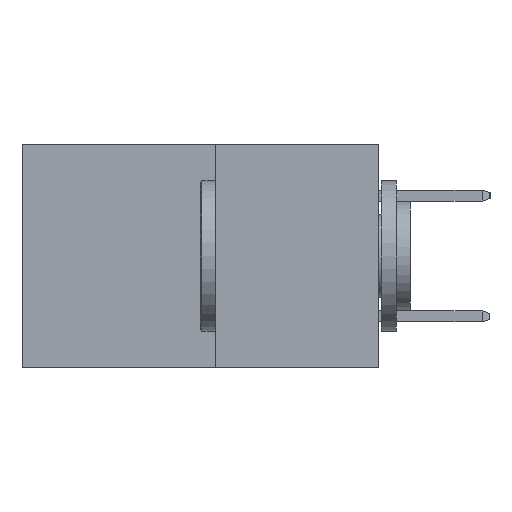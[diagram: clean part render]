
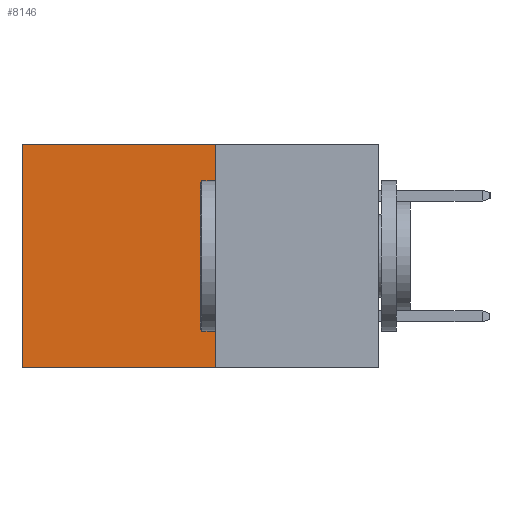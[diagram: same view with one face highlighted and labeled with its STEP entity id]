
A CAD part, left-side view. The second image highlights one B-rep face of the part: STEP entity #8146.
In plain terms, the highlighted planar face has unit normal (-1, 0, 0).
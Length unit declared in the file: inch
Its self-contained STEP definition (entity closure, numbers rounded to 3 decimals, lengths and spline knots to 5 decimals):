
#249 = CARTESIAN_POINT ( 'NONE',  ( 0.277, 0.59, -0.37 ) ) ;
#327 = DIRECTION ( 'NONE',  ( 0., 0., -1. ) ) ;
#389 = EDGE_CURVE ( 'NONE', #13728, #2736, #17457, .T. ) ;
#1051 = DIRECTION ( 'NONE',  ( 0., 1., 0. ) ) ;
#1529 = CARTESIAN_POINT ( 'NONE',  ( 0.277, 0.59, 0. ) ) ;
#1796 = LINE ( 'NONE', #249, #10206 ) ;
#2736 = VERTEX_POINT ( 'NONE', #16507 ) ;
#3475 = FACE_OUTER_BOUND ( 'NONE', #16421, .T. ) ;
#6684 = ORIENTED_EDGE ( 'NONE', *, *, #389, .F. ) ;
#6734 = AXIS2_PLACEMENT_3D ( 'NONE', #14600, #9580, #9412 ) ;
#7220 = DIRECTION ( 'NONE',  ( 0., 1., 0. ) ) ;
#7589 = LINE ( 'NONE', #12164, #19640 ) ;
#8146 = ADVANCED_FACE ( 'NONE', ( #3475 ), #11537, .F. ) ;
#9412 = DIRECTION ( 'NONE',  ( 0., 0., -1. ) ) ;
#9580 = DIRECTION ( 'NONE',  ( 1., 0., 0. ) ) ;
#10144 = CARTESIAN_POINT ( 'NONE',  ( 0.277, 0.59, -0.37 ) ) ;
#10206 = VECTOR ( 'NONE', #327, 39.37008 ) ;
#10734 = DIRECTION ( 'NONE',  ( 0., 0., -1. ) ) ;
#11537 = PLANE ( 'NONE',  #6734 ) ;
#11620 = LINE ( 'NONE', #20886, #19781 ) ;
#12164 = CARTESIAN_POINT ( 'NONE',  ( 0.277, 0.27, -0.37 ) ) ;
#12447 = EDGE_CURVE ( 'NONE', #13728, #13957, #11620, .T. ) ;
#13350 = VERTEX_POINT ( 'NONE', #10144 ) ;
#13728 = VERTEX_POINT ( 'NONE', #16050 ) ;
#13957 = VERTEX_POINT ( 'NONE', #1529 ) ;
#14296 = ORIENTED_EDGE ( 'NONE', *, *, #12447, .T. ) ;
#14600 = CARTESIAN_POINT ( 'NONE',  ( 0.277, 0.27, -0.37 ) ) ;
#15175 = EDGE_CURVE ( 'NONE', #2736, #13350, #7589, .T. ) ;
#15751 = ORIENTED_EDGE ( 'NONE', *, *, #15830, .T. ) ;
#15830 = EDGE_CURVE ( 'NONE', #13957, #13350, #1796, .T. ) ;
#16050 = CARTESIAN_POINT ( 'NONE',  ( 0.277, 0.27, 0. ) ) ;
#16421 = EDGE_LOOP ( 'NONE', ( #15751, #17460, #6684, #14296 ) ) ;
#16507 = CARTESIAN_POINT ( 'NONE',  ( 0.277, 0.27, -0.37 ) ) ;
#17457 = LINE ( 'NONE', #20308, #17965 ) ;
#17460 = ORIENTED_EDGE ( 'NONE', *, *, #15175, .F. ) ;
#17965 = VECTOR ( 'NONE', #10734, 39.37008 ) ;
#19640 = VECTOR ( 'NONE', #7220, 39.37008 ) ;
#19781 = VECTOR ( 'NONE', #1051, 39.37008 ) ;
#20308 = CARTESIAN_POINT ( 'NONE',  ( 0.277, 0.27, -0.37 ) ) ;
#20886 = CARTESIAN_POINT ( 'NONE',  ( 0.277, 0.27, 0. ) ) ;
